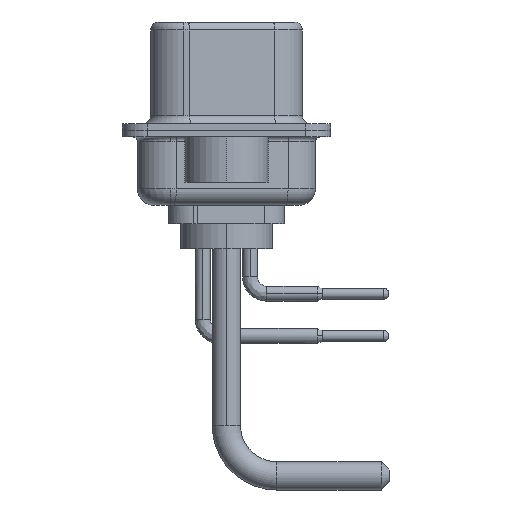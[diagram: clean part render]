
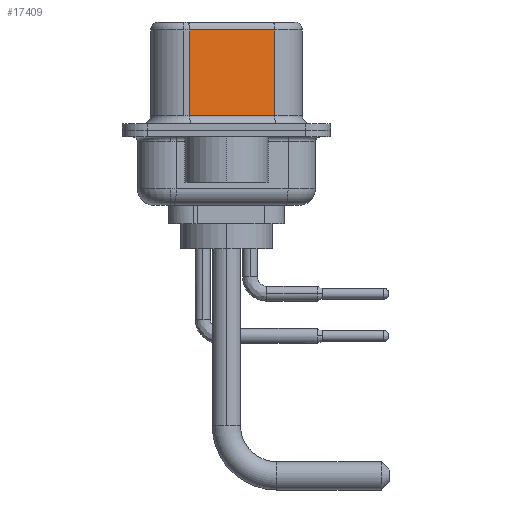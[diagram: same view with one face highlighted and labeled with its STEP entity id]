
A CAD part, left-side view. The second image highlights one B-rep face of the part: STEP entity #17409.
In plain terms, the highlighted planar face has unit normal (-0.985, -0.174, 0).
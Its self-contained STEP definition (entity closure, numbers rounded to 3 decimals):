
#1149 = LINE ( 'NONE', #17003, #14865 ) ;
#1904 = DIRECTION ( 'NONE',  ( 0.174, -0.985, 0. ) ) ;
#2430 = VERTEX_POINT ( 'NONE', #14969 ) ;
#4164 = EDGE_CURVE ( 'NONE', #6803, #14344, #1149, .T. ) ;
#4258 = ORIENTED_EDGE ( 'NONE', *, *, #19132, .T. ) ;
#4485 = CARTESIAN_POINT ( 'NONE',  ( 4.58, -2.897, 6.52 ) ) ;
#5465 = CARTESIAN_POINT ( 'NONE',  ( 4.58, -2.897, 0.9 ) ) ;
#6046 = DIRECTION ( 'NONE',  ( -0.174, 0.985, 0. ) ) ;
#6177 = CARTESIAN_POINT ( 'NONE',  ( 3.68, 2.203, 6.52 ) ) ;
#6698 = CARTESIAN_POINT ( 'NONE',  ( 3.68, 2.203, 6.02 ) ) ;
#6803 = VERTEX_POINT ( 'NONE', #23730 ) ;
#8430 = EDGE_CURVE ( 'NONE', #2430, #14344, #23725, .T. ) ;
#9058 = VECTOR ( 'NONE', #10232, 1000. ) ;
#10232 = DIRECTION ( 'NONE',  ( 0., 0., -1. ) ) ;
#11046 = ORIENTED_EDGE ( 'NONE', *, *, #4164, .F. ) ;
#11399 = VECTOR ( 'NONE', #1904, 1000. ) ;
#11650 = EDGE_CURVE ( 'NONE', #11808, #2430, #23963, .T. ) ;
#11808 = VERTEX_POINT ( 'NONE', #6698 ) ;
#12418 = DIRECTION ( 'NONE',  ( 0.985, 0.174, 0. ) ) ;
#12537 = PLANE ( 'NONE',  #17584 ) ;
#14216 = EDGE_LOOP ( 'NONE', ( #11046, #4258, #20291, #24000 ) ) ;
#14344 = VERTEX_POINT ( 'NONE', #5465 ) ;
#14865 = VECTOR ( 'NONE', #24917, 1000. ) ;
#14969 = CARTESIAN_POINT ( 'NONE',  ( 3.68, 2.203, 0.9 ) ) ;
#15103 = VECTOR ( 'NONE', #24579, 1000. ) ;
#16047 = CARTESIAN_POINT ( 'NONE',  ( 4.58, -2.897, 6.02 ) ) ;
#17003 = CARTESIAN_POINT ( 'NONE',  ( 4.58, -2.897, 6.52 ) ) ;
#17409 = ADVANCED_FACE ( 'NONE', ( #20069 ), #12537, .F. ) ;
#17584 = AXIS2_PLACEMENT_3D ( 'NONE', #4485, #12418, #6046 ) ;
#18114 = LINE ( 'NONE', #16047, #15103 ) ;
#19132 = EDGE_CURVE ( 'NONE', #6803, #11808, #18114, .T. ) ;
#20069 = FACE_OUTER_BOUND ( 'NONE', #14216, .T. ) ;
#20291 = ORIENTED_EDGE ( 'NONE', *, *, #11650, .T. ) ;
#22028 = CARTESIAN_POINT ( 'NONE',  ( 4.58, -2.897, 0.9 ) ) ;
#23725 = LINE ( 'NONE', #22028, #11399 ) ;
#23730 = CARTESIAN_POINT ( 'NONE',  ( 4.58, -2.897, 6.02 ) ) ;
#23963 = LINE ( 'NONE', #6177, #9058 ) ;
#24000 = ORIENTED_EDGE ( 'NONE', *, *, #8430, .T. ) ;
#24579 = DIRECTION ( 'NONE',  ( -0.174, 0.985, 0. ) ) ;
#24917 = DIRECTION ( 'NONE',  ( 0., 0., -1. ) ) ;
